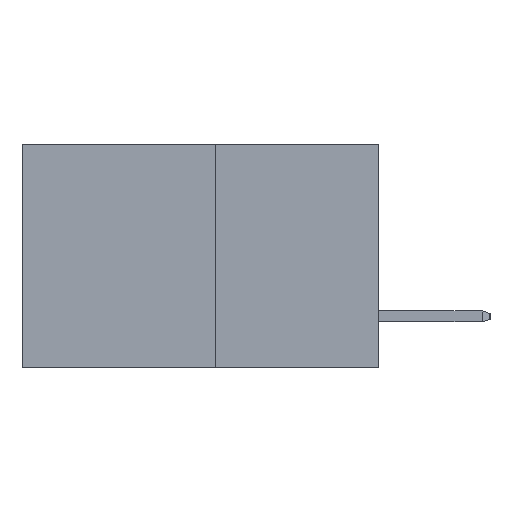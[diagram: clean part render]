
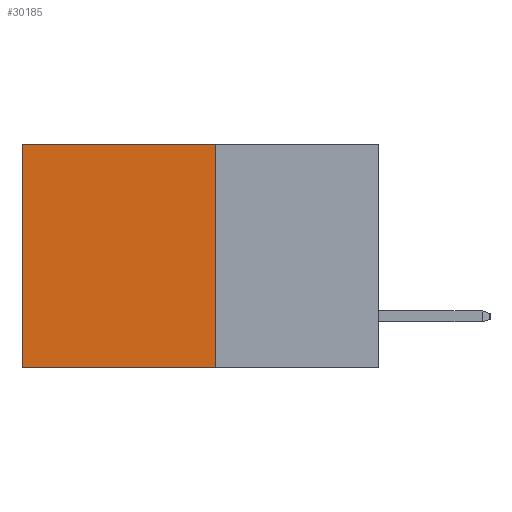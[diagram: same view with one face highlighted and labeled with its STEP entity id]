
A CAD part, left-side view. The second image highlights one B-rep face of the part: STEP entity #30185.
In plain terms, the highlighted planar face has unit normal (-1, 0, 0).
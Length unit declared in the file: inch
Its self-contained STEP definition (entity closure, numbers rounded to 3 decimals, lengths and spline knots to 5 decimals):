
#907 = ORIENTED_EDGE ( 'NONE', *, *, #22404, .T. ) ;
#2807 = CARTESIAN_POINT ( 'NONE',  ( 0.277, 0.27, -0.37 ) ) ;
#5578 = VECTOR ( 'NONE', #29968, 39.37008 ) ;
#7524 = VECTOR ( 'NONE', #19961, 39.37008 ) ;
#8045 = ORIENTED_EDGE ( 'NONE', *, *, #29992, .F. ) ;
#8255 = AXIS2_PLACEMENT_3D ( 'NONE', #20291, #13220, #29514 ) ;
#9651 = VERTEX_POINT ( 'NONE', #15536 ) ;
#11522 = VERTEX_POINT ( 'NONE', #15746 ) ;
#12223 = VECTOR ( 'NONE', #22856, 39.37008 ) ;
#13220 = DIRECTION ( 'NONE',  ( 1., 0., 0. ) ) ;
#13335 = CARTESIAN_POINT ( 'NONE',  ( 0.277, 0.59, -0.37 ) ) ;
#13858 = LINE ( 'NONE', #17577, #7524 ) ;
#14302 = CARTESIAN_POINT ( 'NONE',  ( 0.277, 0.59, 0. ) ) ;
#14508 = CARTESIAN_POINT ( 'NONE',  ( 0.277, 0.27, -0.37 ) ) ;
#15536 = CARTESIAN_POINT ( 'NONE',  ( 0.277, 0.27, 0. ) ) ;
#15746 = CARTESIAN_POINT ( 'NONE',  ( 0.277, 0.59, -0.37 ) ) ;
#16083 = CARTESIAN_POINT ( 'NONE',  ( 0.277, 0.27, 0. ) ) ;
#17577 = CARTESIAN_POINT ( 'NONE',  ( 0.277, 0.27, -0.37 ) ) ;
#18217 = LINE ( 'NONE', #16083, #5578 ) ;
#18543 = LINE ( 'NONE', #13335, #12223 ) ;
#18928 = VECTOR ( 'NONE', #21844, 39.37008 ) ;
#19340 = VERTEX_POINT ( 'NONE', #14508 ) ;
#19961 = DIRECTION ( 'NONE',  ( 0., 0., -1. ) ) ;
#20246 = EDGE_CURVE ( 'NONE', #9651, #19340, #13858, .T. ) ;
#20291 = CARTESIAN_POINT ( 'NONE',  ( 0.277, 0.27, -0.37 ) ) ;
#21217 = ORIENTED_EDGE ( 'NONE', *, *, #21816, .T. ) ;
#21816 = EDGE_CURVE ( 'NONE', #9651, #26499, #18217, .T. ) ;
#21844 = DIRECTION ( 'NONE',  ( 0., 1., 0. ) ) ;
#22404 = EDGE_CURVE ( 'NONE', #26499, #11522, #18543, .T. ) ;
#22856 = DIRECTION ( 'NONE',  ( 0., 0., -1. ) ) ;
#24794 = EDGE_LOOP ( 'NONE', ( #907, #8045, #28615, #21217 ) ) ;
#25113 = LINE ( 'NONE', #2807, #18928 ) ;
#25448 = FACE_OUTER_BOUND ( 'NONE', #24794, .T. ) ;
#26499 = VERTEX_POINT ( 'NONE', #14302 ) ;
#27217 = PLANE ( 'NONE',  #8255 ) ;
#28615 = ORIENTED_EDGE ( 'NONE', *, *, #20246, .F. ) ;
#29514 = DIRECTION ( 'NONE',  ( 0., 0., -1. ) ) ;
#29968 = DIRECTION ( 'NONE',  ( 0., 1., 0. ) ) ;
#29992 = EDGE_CURVE ( 'NONE', #19340, #11522, #25113, .T. ) ;
#30185 = ADVANCED_FACE ( 'NONE', ( #25448 ), #27217, .F. ) ;
